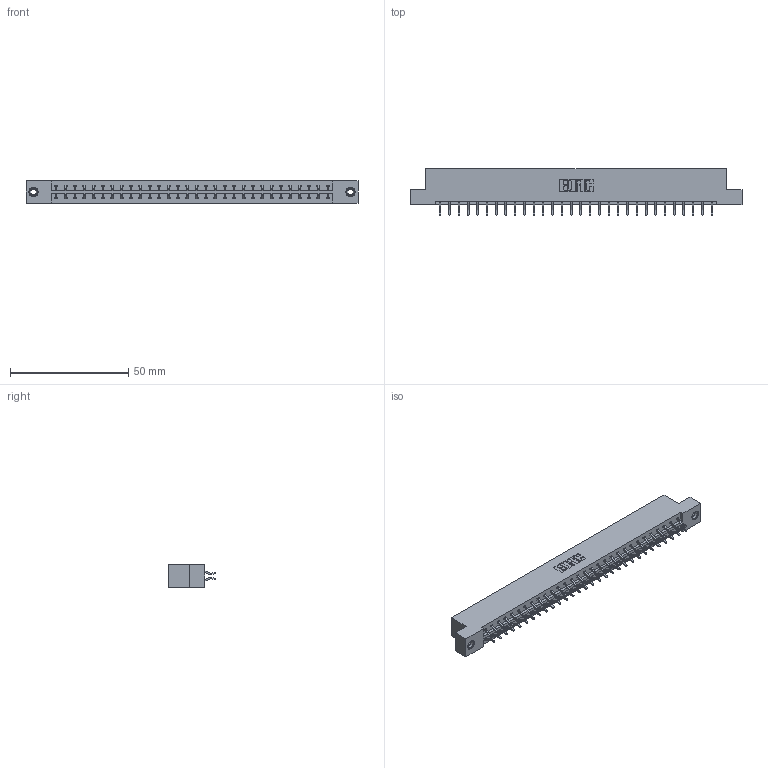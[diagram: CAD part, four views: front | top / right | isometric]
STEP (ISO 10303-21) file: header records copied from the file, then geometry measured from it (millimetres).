
FILE_DESCRIPTION (( 'STEP AP203' ), '1' );
FILE_NAME ('833-060-556-208.STEP', '2020-06-05T04:33:09', ( '' ), ( '' ), 'SwSTEP 2.0', 'SolidWorks 2020', '' );
FILE_SCHEMA (( 'CONFIG_CONTROL_DESIGN' ));
Length unit declared in the file: inch
Products named in the file (4): 833-060-556-208; 833 Part_Flush - .156 Dia - TI; 345-250-001_345-250-003-102; 345-292-001_556 Tail
Assembly tree (63 placements, depth 2):
  833-060-556-208
    833 Part_Flush - .156 Dia - TI
    345-292-001_556 Tail  x60
    345-250-001_345-250-003-102  x2
Bounding box: 140.41 x 19.57 x 9.4 mm (x, y, z)
Volume: 14214.1 mm3; surface area: 16638.2 mm2
Topology: 63 solids, 63 shells, 3654 faces, 10827 edges, 7130 vertices
Faces by surface type: plane 2502, cylinder 1136, cone 12, torus 4
Entity records: 22258 total; most frequent: CARTESIAN_POINT 3701, ORIENTED_EDGE 3618, DIRECTION 3203, EDGE_CURVE 1809, LINE 1653, VECTOR 1653, VERTEX_POINT 1200, AXIS2_PLACEMENT_3D 775
